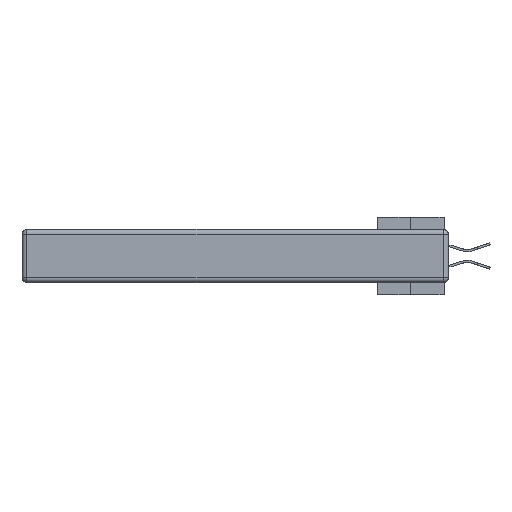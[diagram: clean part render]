
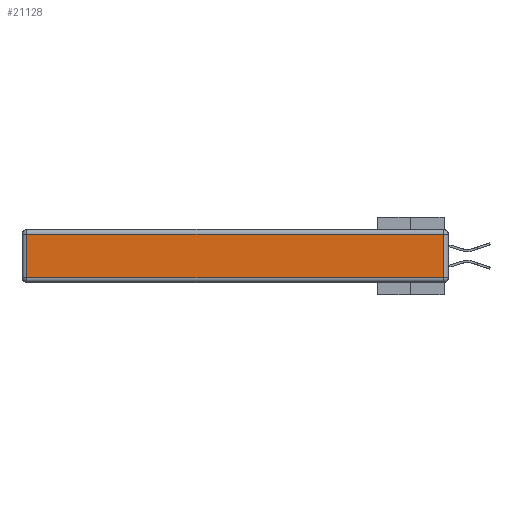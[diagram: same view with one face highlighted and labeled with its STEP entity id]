
A CAD part, left-side view. The second image highlights one B-rep face of the part: STEP entity #21128.
In plain terms, the highlighted planar face has unit normal (-1, 0, 0).
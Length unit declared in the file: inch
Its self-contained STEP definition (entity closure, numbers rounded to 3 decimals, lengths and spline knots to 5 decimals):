
#2800 = EDGE_CURVE ( 'NONE', #13774, #7583, #24465, .T. ) ;
#4237 = EDGE_CURVE ( 'NONE', #7583, #12005, #29459, .T. ) ;
#6196 = CARTESIAN_POINT ( 'NONE',  ( 0., 2.72, -0.343 ) ) ;
#7352 = CARTESIAN_POINT ( 'NONE',  ( 0., 0.03, -0.343 ) ) ;
#7583 = VERTEX_POINT ( 'NONE', #14628 ) ;
#7685 = LINE ( 'NONE', #7352, #36344 ) ;
#8774 = ORIENTED_EDGE ( 'NONE', *, *, #2800, .T. ) ;
#9454 = DIRECTION ( 'NONE',  ( 0., -1., 0. ) ) ;
#9972 = VERTEX_POINT ( 'NONE', #35048 ) ;
#10556 = DIRECTION ( 'NONE',  ( 0., 0., 1. ) ) ;
#12005 = VERTEX_POINT ( 'NONE', #34675 ) ;
#12131 = EDGE_CURVE ( 'NONE', #12005, #9972, #18896, .T. ) ;
#12676 = CARTESIAN_POINT ( 'NONE',  ( 0., 2.75, -0.03 ) ) ;
#13774 = VERTEX_POINT ( 'NONE', #14997 ) ;
#14085 = CARTESIAN_POINT ( 'NONE',  ( 0., 0., -0.343 ) ) ;
#14628 = CARTESIAN_POINT ( 'NONE',  ( 0., 2.72, -0.03 ) ) ;
#14997 = CARTESIAN_POINT ( 'NONE',  ( 0., 0.03, -0.03 ) ) ;
#15605 = VECTOR ( 'NONE', #31613, 39.37008 ) ;
#16601 = ORIENTED_EDGE ( 'NONE', *, *, #22543, .T. ) ;
#18896 = LINE ( 'NONE', #28528, #37268 ) ;
#21128 = ADVANCED_FACE ( 'NONE', ( #21528 ), #30580, .T. ) ;
#21528 = FACE_OUTER_BOUND ( 'NONE', #30712, .T. ) ;
#22373 = DIRECTION ( 'NONE',  ( 0., 1., 0. ) ) ;
#22543 = EDGE_CURVE ( 'NONE', #9972, #13774, #7685, .T. ) ;
#23753 = DIRECTION ( 'NONE',  ( -1., 0., 0. ) ) ;
#24465 = LINE ( 'NONE', #12676, #40412 ) ;
#28528 = CARTESIAN_POINT ( 'NONE',  ( 0., 0., -0.313 ) ) ;
#28621 = ORIENTED_EDGE ( 'NONE', *, *, #4237, .T. ) ;
#29459 = LINE ( 'NONE', #6196, #15605 ) ;
#30580 = PLANE ( 'NONE',  #34233 ) ;
#30712 = EDGE_LOOP ( 'NONE', ( #40183, #16601, #8774, #28621 ) ) ;
#31613 = DIRECTION ( 'NONE',  ( 0., 0., -1. ) ) ;
#34233 = AXIS2_PLACEMENT_3D ( 'NONE', #14085, #23753, #36746 ) ;
#34675 = CARTESIAN_POINT ( 'NONE',  ( 0., 2.72, -0.313 ) ) ;
#35048 = CARTESIAN_POINT ( 'NONE',  ( 0., 0.03, -0.313 ) ) ;
#36344 = VECTOR ( 'NONE', #10556, 39.37008 ) ;
#36746 = DIRECTION ( 'NONE',  ( 0., 0., 1. ) ) ;
#37268 = VECTOR ( 'NONE', #9454, 39.37008 ) ;
#40183 = ORIENTED_EDGE ( 'NONE', *, *, #12131, .T. ) ;
#40412 = VECTOR ( 'NONE', #22373, 39.37008 ) ;
